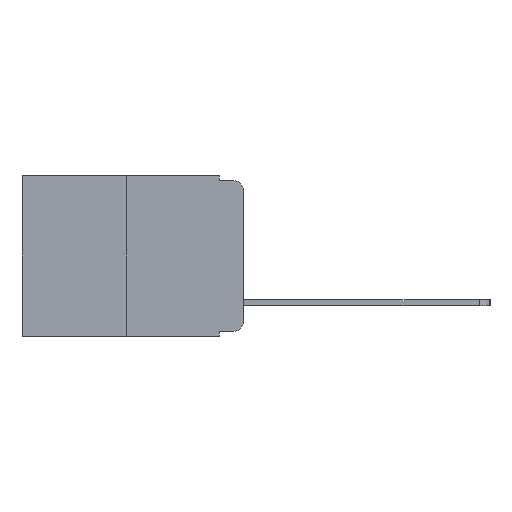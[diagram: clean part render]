
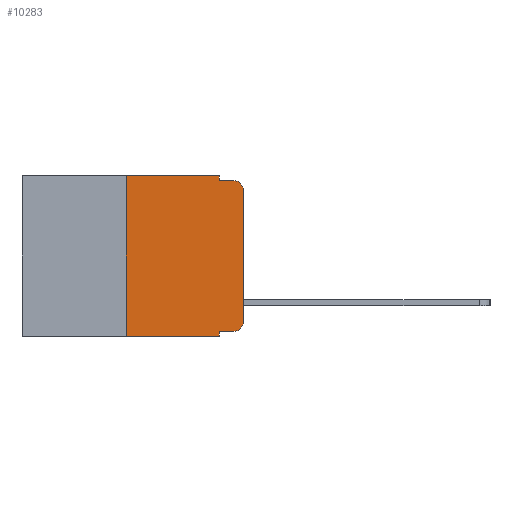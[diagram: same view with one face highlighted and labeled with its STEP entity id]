
A CAD part, left-side view. The second image highlights one B-rep face of the part: STEP entity #10283.
In plain terms, the highlighted planar face has unit normal (-1, 0, 0).
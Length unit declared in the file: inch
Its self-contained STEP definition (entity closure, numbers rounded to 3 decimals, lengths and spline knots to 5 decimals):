
#539 = CARTESIAN_POINT ( 'NONE',  ( 0., 0., 0. ) ) ;
#840 = VECTOR ( 'NONE', #9758, 39.37008 ) ;
#921 = VERTEX_POINT ( 'NONE', #16017 ) ;
#1149 = DIRECTION ( 'NONE',  ( 0., 0., 1. ) ) ;
#1182 = ORIENTED_EDGE ( 'NONE', *, *, #13987, .F. ) ;
#1544 = CARTESIAN_POINT ( 'NONE',  ( 0., 0.02, -0.333 ) ) ;
#1602 = FACE_OUTER_BOUND ( 'NONE', #3396, .T. ) ;
#1822 = ORIENTED_EDGE ( 'NONE', *, *, #11134, .F. ) ;
#1914 = CIRCLE ( 'NONE', #13823, 0.02 ) ;
#1977 = ORIENTED_EDGE ( 'NONE', *, *, #9145, .F. ) ;
#2363 = CARTESIAN_POINT ( 'NONE',  ( 0., 0.473, 0. ) ) ;
#2676 = EDGE_CURVE ( 'NONE', #921, #6049, #12929, .T. ) ;
#2685 = EDGE_CURVE ( 'NONE', #14761, #13676, #5921, .T. ) ;
#2816 = CARTESIAN_POINT ( 'NONE',  ( 0., 0.02, -0.313 ) ) ;
#3298 = LINE ( 'NONE', #5155, #6332 ) ;
#3371 = PLANE ( 'NONE',  #12062 ) ;
#3396 = EDGE_LOOP ( 'NONE', ( #8680, #9826, #1182, #3620, #13324, #1822, #12355, #1977, #3492, #15734 ) ) ;
#3492 = ORIENTED_EDGE ( 'NONE', *, *, #2676, .T. ) ;
#3620 = ORIENTED_EDGE ( 'NONE', *, *, #2685, .F. ) ;
#3664 = VECTOR ( 'NONE', #6240, 39.37008 ) ;
#3930 = CARTESIAN_POINT ( 'NONE',  ( 0., 0.051, 0. ) ) ;
#4127 = DIRECTION ( 'NONE',  ( 0., 0., -1. ) ) ;
#4480 = LINE ( 'NONE', #539, #840 ) ;
#4498 = LINE ( 'NONE', #4957, #3664 ) ;
#4562 = CARTESIAN_POINT ( 'NONE',  ( 0., 0.051, -0.01 ) ) ;
#4697 = DIRECTION ( 'NONE',  ( 1., 0., 0. ) ) ;
#4826 = VECTOR ( 'NONE', #6289, 39.37008 ) ;
#4957 = CARTESIAN_POINT ( 'NONE',  ( 0., 0.473, -0.343 ) ) ;
#5101 = CARTESIAN_POINT ( 'NONE',  ( 0., 0.051, -0.01 ) ) ;
#5155 = CARTESIAN_POINT ( 'NONE',  ( 0., 0.25, 0. ) ) ;
#5259 = VECTOR ( 'NONE', #14984, 39.37008 ) ;
#5533 = VECTOR ( 'NONE', #15098, 39.37008 ) ;
#5575 = EDGE_CURVE ( 'NONE', #8319, #12194, #1914, .T. ) ;
#5635 = DIRECTION ( 'NONE',  ( -1., 0., 0. ) ) ;
#5921 = LINE ( 'NONE', #15042, #5533 ) ;
#6049 = VERTEX_POINT ( 'NONE', #1544 ) ;
#6240 = DIRECTION ( 'NONE',  ( 0., -1., 0. ) ) ;
#6289 = DIRECTION ( 'NONE',  ( 0., -1., 0. ) ) ;
#6325 = VECTOR ( 'NONE', #10224, 39.37008 ) ;
#6332 = VECTOR ( 'NONE', #1149, 39.37008 ) ;
#6456 = EDGE_CURVE ( 'NONE', #15007, #14761, #8209, .T. ) ;
#8209 = LINE ( 'NONE', #2363, #4826 ) ;
#8319 = VERTEX_POINT ( 'NONE', #11187 ) ;
#8680 = ORIENTED_EDGE ( 'NONE', *, *, #15861, .T. ) ;
#9081 = LINE ( 'NONE', #5101, #5259 ) ;
#9145 = EDGE_CURVE ( 'NONE', #921, #10489, #16354, .T. ) ;
#9521 = CIRCLE ( 'NONE', #14551, 0.02 ) ;
#9758 = DIRECTION ( 'NONE',  ( 0., 0., 1. ) ) ;
#9776 = CARTESIAN_POINT ( 'NONE',  ( 0., 0.473, 0. ) ) ;
#9826 = ORIENTED_EDGE ( 'NONE', *, *, #5575, .T. ) ;
#10010 = VECTOR ( 'NONE', #12717, 39.37008 ) ;
#10224 = DIRECTION ( 'NONE',  ( 0., -1., 0. ) ) ;
#10283 = ADVANCED_FACE ( 'NONE', ( #1602 ), #3371, .F. ) ;
#10489 = VERTEX_POINT ( 'NONE', #16106 ) ;
#11134 = EDGE_CURVE ( 'NONE', #16043, #15007, #3298, .T. ) ;
#11187 = CARTESIAN_POINT ( 'NONE',  ( 0., 0., -0.03 ) ) ;
#11302 = CARTESIAN_POINT ( 'NONE',  ( 0., 0.25, -0.343 ) ) ;
#11697 = DIRECTION ( 'NONE',  ( -1., 0., 0. ) ) ;
#11923 = EDGE_CURVE ( 'NONE', #6049, #15134, #9521, .T. ) ;
#12062 = AXIS2_PLACEMENT_3D ( 'NONE', #9776, #4697, #13392 ) ;
#12176 = CARTESIAN_POINT ( 'NONE',  ( 0., 0.02, -0.01 ) ) ;
#12194 = VERTEX_POINT ( 'NONE', #12176 ) ;
#12355 = ORIENTED_EDGE ( 'NONE', *, *, #15418, .T. ) ;
#12717 = DIRECTION ( 'NONE',  ( 0., 0., -1. ) ) ;
#12929 = LINE ( 'NONE', #15854, #6325 ) ;
#13091 = CARTESIAN_POINT ( 'NONE',  ( 0., 0.02, -0.03 ) ) ;
#13238 = CARTESIAN_POINT ( 'NONE',  ( 0., 0., -0.313 ) ) ;
#13324 = ORIENTED_EDGE ( 'NONE', *, *, #6456, .F. ) ;
#13392 = DIRECTION ( 'NONE',  ( 0., 0., -1. ) ) ;
#13676 = VERTEX_POINT ( 'NONE', #4562 ) ;
#13823 = AXIS2_PLACEMENT_3D ( 'NONE', #13091, #5635, #14260 ) ;
#13987 = EDGE_CURVE ( 'NONE', #13676, #12194, #9081, .T. ) ;
#14211 = CARTESIAN_POINT ( 'NONE',  ( 0., 0.25, 0. ) ) ;
#14260 = DIRECTION ( 'NONE',  ( 0., 0., -1. ) ) ;
#14551 = AXIS2_PLACEMENT_3D ( 'NONE', #2816, #11697, #4127 ) ;
#14761 = VERTEX_POINT ( 'NONE', #16266 ) ;
#14984 = DIRECTION ( 'NONE',  ( 0., -1., 0. ) ) ;
#15007 = VERTEX_POINT ( 'NONE', #14211 ) ;
#15042 = CARTESIAN_POINT ( 'NONE',  ( 0., 0.051, 0. ) ) ;
#15098 = DIRECTION ( 'NONE',  ( 0., 0., -1. ) ) ;
#15134 = VERTEX_POINT ( 'NONE', #13238 ) ;
#15418 = EDGE_CURVE ( 'NONE', #16043, #10489, #4498, .T. ) ;
#15734 = ORIENTED_EDGE ( 'NONE', *, *, #11923, .T. ) ;
#15854 = CARTESIAN_POINT ( 'NONE',  ( 0., 0.051, -0.333 ) ) ;
#15861 = EDGE_CURVE ( 'NONE', #15134, #8319, #4480, .T. ) ;
#16017 = CARTESIAN_POINT ( 'NONE',  ( 0., 0.051, -0.333 ) ) ;
#16043 = VERTEX_POINT ( 'NONE', #11302 ) ;
#16106 = CARTESIAN_POINT ( 'NONE',  ( 0., 0.051, -0.343 ) ) ;
#16266 = CARTESIAN_POINT ( 'NONE',  ( 0., 0.051, 0. ) ) ;
#16354 = LINE ( 'NONE', #3930, #10010 ) ;
